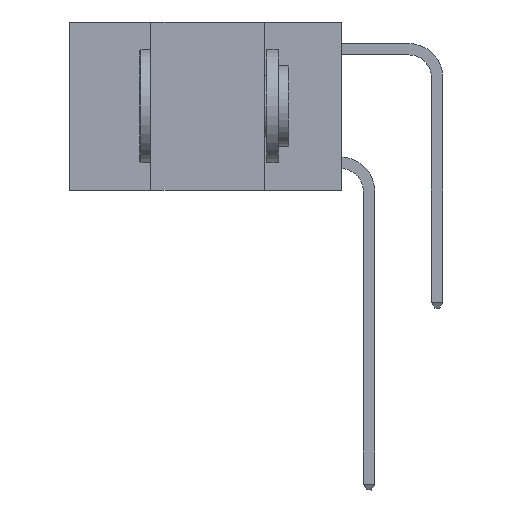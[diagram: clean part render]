
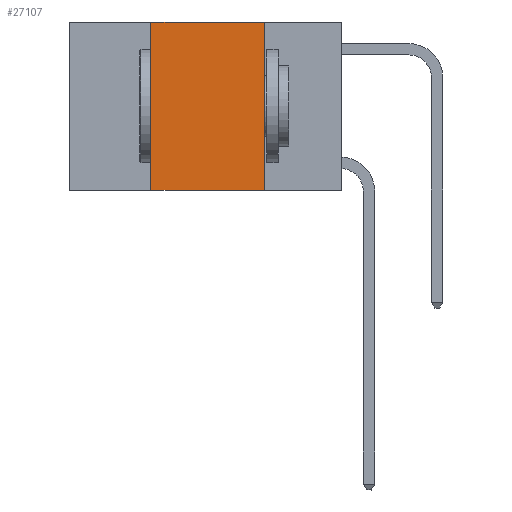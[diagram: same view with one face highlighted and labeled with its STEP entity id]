
A CAD part, left-side view. The second image highlights one B-rep face of the part: STEP entity #27107.
In plain terms, the highlighted planar face has unit normal (-1, 0, 0).
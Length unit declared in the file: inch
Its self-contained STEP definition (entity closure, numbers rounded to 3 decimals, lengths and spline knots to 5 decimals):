
#47 = CARTESIAN_POINT ( 'NONE',  ( 0., 0.6, 0. ) ) ;
#923 = CARTESIAN_POINT ( 'NONE',  ( 0., 0.42, 0. ) ) ;
#2605 = DIRECTION ( 'NONE',  ( 1., 0., 0. ) ) ;
#3240 = EDGE_LOOP ( 'NONE', ( #12513, #21676, #7500, #16990 ) ) ;
#5502 = CARTESIAN_POINT ( 'NONE',  ( 0., 0.17, 0. ) ) ;
#6646 = CARTESIAN_POINT ( 'NONE',  ( 0., 0.42, 0. ) ) ;
#7207 = DIRECTION ( 'NONE',  ( 0., -1., 0. ) ) ;
#7286 = LINE ( 'NONE', #5502, #15643 ) ;
#7500 = ORIENTED_EDGE ( 'NONE', *, *, #13593, .F. ) ;
#9144 = VECTOR ( 'NONE', #15729, 39.37008 ) ;
#11625 = CARTESIAN_POINT ( 'NONE',  ( 0., 0.17, 0. ) ) ;
#12513 = ORIENTED_EDGE ( 'NONE', *, *, #23684, .F. ) ;
#13593 = EDGE_CURVE ( 'NONE', #25492, #26349, #22414, .T. ) ;
#13771 = CARTESIAN_POINT ( 'NONE',  ( 0., 0.17, -0.37 ) ) ;
#15274 = DIRECTION ( 'NONE',  ( 0., -1., 0. ) ) ;
#15643 = VECTOR ( 'NONE', #25427, 39.37008 ) ;
#15729 = DIRECTION ( 'NONE',  ( 0., 0., 1. ) ) ;
#15784 = VERTEX_POINT ( 'NONE', #11625 ) ;
#16990 = ORIENTED_EDGE ( 'NONE', *, *, #27303, .T. ) ;
#17142 = AXIS2_PLACEMENT_3D ( 'NONE', #20774, #2605, #21213 ) ;
#17256 = VERTEX_POINT ( 'NONE', #13771 ) ;
#17258 = EDGE_CURVE ( 'NONE', #26349, #15784, #23277, .T. ) ;
#17784 = VECTOR ( 'NONE', #7207, 39.37008 ) ;
#19615 = CARTESIAN_POINT ( 'NONE',  ( 0., 0.42, -0.37 ) ) ;
#19728 = LINE ( 'NONE', #26998, #23296 ) ;
#20774 = CARTESIAN_POINT ( 'NONE',  ( 0., 0.6, 0. ) ) ;
#20916 = FACE_OUTER_BOUND ( 'NONE', #3240, .T. ) ;
#21213 = DIRECTION ( 'NONE',  ( 0., 0., -1. ) ) ;
#21676 = ORIENTED_EDGE ( 'NONE', *, *, #17258, .F. ) ;
#22414 = LINE ( 'NONE', #6646, #9144 ) ;
#22998 = PLANE ( 'NONE',  #17142 ) ;
#23277 = LINE ( 'NONE', #47, #17784 ) ;
#23296 = VECTOR ( 'NONE', #15274, 39.37008 ) ;
#23684 = EDGE_CURVE ( 'NONE', #15784, #17256, #7286, .T. ) ;
#25427 = DIRECTION ( 'NONE',  ( 0., 0., -1. ) ) ;
#25492 = VERTEX_POINT ( 'NONE', #19615 ) ;
#26349 = VERTEX_POINT ( 'NONE', #923 ) ;
#26998 = CARTESIAN_POINT ( 'NONE',  ( 0., 0.6, -0.37 ) ) ;
#27107 = ADVANCED_FACE ( 'NONE', ( #20916 ), #22998, .F. ) ;
#27303 = EDGE_CURVE ( 'NONE', #25492, #17256, #19728, .T. ) ;
